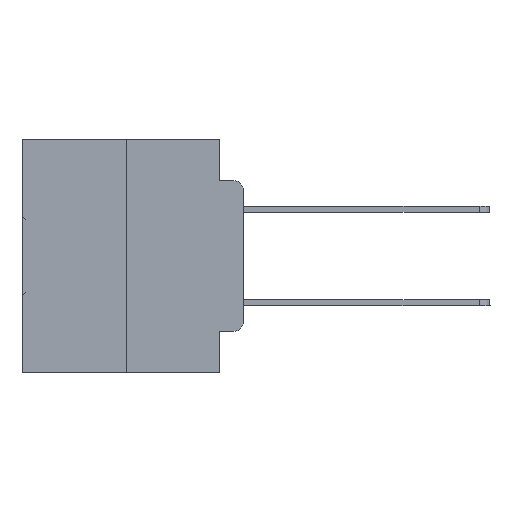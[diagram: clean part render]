
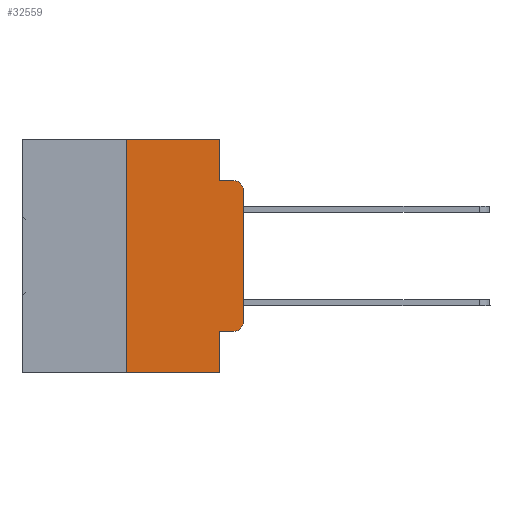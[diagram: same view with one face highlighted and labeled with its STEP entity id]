
A CAD part, left-side view. The second image highlights one B-rep face of the part: STEP entity #32559.
In plain terms, the highlighted planar face has unit normal (-1, 0, 0).
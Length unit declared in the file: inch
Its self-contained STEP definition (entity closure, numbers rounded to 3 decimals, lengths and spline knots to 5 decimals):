
#481 = EDGE_LOOP ( 'NONE', ( #11133, #15310, #32565, #15936, #12223, #24133, #1684, #28041, #7674, #5972 ) ) ;
#1031 = PLANE ( 'NONE',  #22912 ) ;
#1207 = CARTESIAN_POINT ( 'NONE',  ( 0., 0.473, 0. ) ) ;
#1563 = DIRECTION ( 'NONE',  ( 0., 0., 1. ) ) ;
#1617 = CARTESIAN_POINT ( 'NONE',  ( 0., 0., -0.1085 ) ) ;
#1647 = VERTEX_POINT ( 'NONE', #5030 ) ;
#1684 = ORIENTED_EDGE ( 'NONE', *, *, #3612, .T. ) ;
#2178 = DIRECTION ( 'NONE',  ( 0., -1., 0. ) ) ;
#3182 = CARTESIAN_POINT ( 'NONE',  ( 0., 0.051, -0.0885 ) ) ;
#3349 = DIRECTION ( 'NONE',  ( 0., -1., 0. ) ) ;
#3551 = DIRECTION ( 'NONE',  ( 0., 0., -1. ) ) ;
#3612 = EDGE_CURVE ( 'NONE', #16235, #12690, #18830, .T. ) ;
#5030 = CARTESIAN_POINT ( 'NONE',  ( 0., 0.051, -0.4115 ) ) ;
#5116 = DIRECTION ( 'NONE',  ( 0., -1., 0. ) ) ;
#5165 = LINE ( 'NONE', #18966, #12018 ) ;
#5658 = VECTOR ( 'NONE', #34617, 39.37008 ) ;
#5742 = CARTESIAN_POINT ( 'NONE',  ( 0., 0.02, -0.3915 ) ) ;
#5972 = ORIENTED_EDGE ( 'NONE', *, *, #33330, .T. ) ;
#6468 = CARTESIAN_POINT ( 'NONE',  ( 0., 0.02, -0.4115 ) ) ;
#7674 = ORIENTED_EDGE ( 'NONE', *, *, #11654, .T. ) ;
#8081 = VECTOR ( 'NONE', #23141, 39.37008 ) ;
#8140 = VERTEX_POINT ( 'NONE', #1617 ) ;
#8765 = VERTEX_POINT ( 'NONE', #32740 ) ;
#10099 = VERTEX_POINT ( 'NONE', #18032 ) ;
#10352 = LINE ( 'NONE', #13580, #5658 ) ;
#10730 = CARTESIAN_POINT ( 'NONE',  ( 0., 0.473, -0.5 ) ) ;
#10944 = CARTESIAN_POINT ( 'NONE',  ( 0., 0.25, 0. ) ) ;
#11133 = ORIENTED_EDGE ( 'NONE', *, *, #18644, .T. ) ;
#11654 = EDGE_CURVE ( 'NONE', #1647, #30310, #10352, .T. ) ;
#11745 = LINE ( 'NONE', #22737, #24690 ) ;
#12018 = VECTOR ( 'NONE', #13566, 39.37008 ) ;
#12223 = ORIENTED_EDGE ( 'NONE', *, *, #29640, .F. ) ;
#12690 = VERTEX_POINT ( 'NONE', #30703 ) ;
#13239 = EDGE_CURVE ( 'NONE', #34537, #8765, #21541, .T. ) ;
#13566 = DIRECTION ( 'NONE',  ( 0., 0., 1. ) ) ;
#13580 = CARTESIAN_POINT ( 'NONE',  ( 0., 0.051, -0.4115 ) ) ;
#14994 = DIRECTION ( 'NONE',  ( 1., 0., 0. ) ) ;
#15310 = ORIENTED_EDGE ( 'NONE', *, *, #22808, .T. ) ;
#15936 = ORIENTED_EDGE ( 'NONE', *, *, #17646, .F. ) ;
#16235 = VERTEX_POINT ( 'NONE', #16257 ) ;
#16257 = CARTESIAN_POINT ( 'NONE',  ( 0., 0.25, -0.5 ) ) ;
#16655 = DIRECTION ( 'NONE',  ( -1., 0., 0. ) ) ;
#16792 = AXIS2_PLACEMENT_3D ( 'NONE', #16934, #25045, #33292 ) ;
#16934 = CARTESIAN_POINT ( 'NONE',  ( 0., 0.02, -0.1085 ) ) ;
#17646 = EDGE_CURVE ( 'NONE', #25907, #34537, #23746, .T. ) ;
#17798 = AXIS2_PLACEMENT_3D ( 'NONE', #5742, #16655, #27630 ) ;
#18032 = CARTESIAN_POINT ( 'NONE',  ( 0., 0., -0.3915 ) ) ;
#18504 = CIRCLE ( 'NONE', #16792, 0.02 ) ;
#18644 = EDGE_CURVE ( 'NONE', #10099, #8140, #5165, .T. ) ;
#18830 = LINE ( 'NONE', #10730, #24860 ) ;
#18917 = LINE ( 'NONE', #34893, #33097 ) ;
#18966 = CARTESIAN_POINT ( 'NONE',  ( 0., 0., 0. ) ) ;
#20079 = EDGE_CURVE ( 'NONE', #16235, #30271, #11745, .T. ) ;
#20577 = CARTESIAN_POINT ( 'NONE',  ( 0., 0.051, 0. ) ) ;
#20854 = EDGE_CURVE ( 'NONE', #1647, #12690, #28511, .T. ) ;
#21541 = LINE ( 'NONE', #3182, #22350 ) ;
#22350 = VECTOR ( 'NONE', #3349, 39.37008 ) ;
#22737 = CARTESIAN_POINT ( 'NONE',  ( 0., 0.25, 0. ) ) ;
#22808 = EDGE_CURVE ( 'NONE', #8140, #8765, #18504, .T. ) ;
#22912 = AXIS2_PLACEMENT_3D ( 'NONE', #1207, #14994, #3551 ) ;
#23141 = DIRECTION ( 'NONE',  ( 0., 0., -1. ) ) ;
#23746 = LINE ( 'NONE', #31823, #33795 ) ;
#24133 = ORIENTED_EDGE ( 'NONE', *, *, #20079, .F. ) ;
#24690 = VECTOR ( 'NONE', #1563, 39.37008 ) ;
#24860 = VECTOR ( 'NONE', #2178, 39.37008 ) ;
#25045 = DIRECTION ( 'NONE',  ( -1., 0., 0. ) ) ;
#25907 = VERTEX_POINT ( 'NONE', #20577 ) ;
#26179 = CARTESIAN_POINT ( 'NONE',  ( 0., 0.051, 0. ) ) ;
#26621 = FACE_OUTER_BOUND ( 'NONE', #481, .T. ) ;
#26955 = DIRECTION ( 'NONE',  ( 0., 0., -1. ) ) ;
#27630 = DIRECTION ( 'NONE',  ( 0., 0., -1. ) ) ;
#28041 = ORIENTED_EDGE ( 'NONE', *, *, #20854, .F. ) ;
#28511 = LINE ( 'NONE', #26179, #8081 ) ;
#29275 = CIRCLE ( 'NONE', #17798, 0.02 ) ;
#29640 = EDGE_CURVE ( 'NONE', #30271, #25907, #18917, .T. ) ;
#30271 = VERTEX_POINT ( 'NONE', #10944 ) ;
#30310 = VERTEX_POINT ( 'NONE', #6468 ) ;
#30703 = CARTESIAN_POINT ( 'NONE',  ( 0., 0.051, -0.5 ) ) ;
#31823 = CARTESIAN_POINT ( 'NONE',  ( 0., 0.051, 0. ) ) ;
#32282 = CARTESIAN_POINT ( 'NONE',  ( 0., 0.051, -0.0885 ) ) ;
#32559 = ADVANCED_FACE ( 'NONE', ( #26621 ), #1031, .F. ) ;
#32565 = ORIENTED_EDGE ( 'NONE', *, *, #13239, .F. ) ;
#32740 = CARTESIAN_POINT ( 'NONE',  ( 0., 0.02, -0.0885 ) ) ;
#33097 = VECTOR ( 'NONE', #5116, 39.37008 ) ;
#33292 = DIRECTION ( 'NONE',  ( 0., 0., -1. ) ) ;
#33330 = EDGE_CURVE ( 'NONE', #30310, #10099, #29275, .T. ) ;
#33795 = VECTOR ( 'NONE', #26955, 39.37008 ) ;
#34537 = VERTEX_POINT ( 'NONE', #32282 ) ;
#34617 = DIRECTION ( 'NONE',  ( 0., -1., 0. ) ) ;
#34893 = CARTESIAN_POINT ( 'NONE',  ( 0., 0.473, 0. ) ) ;
